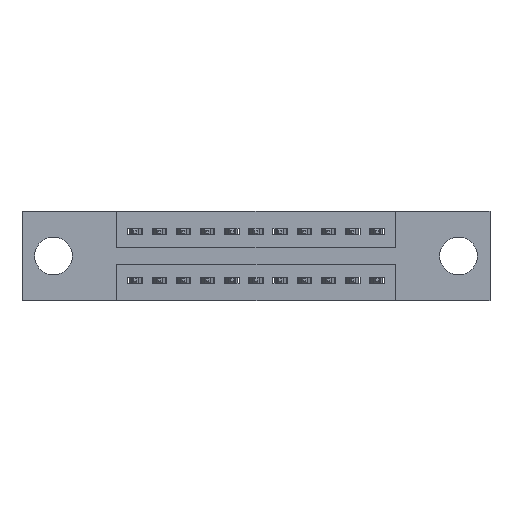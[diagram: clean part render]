
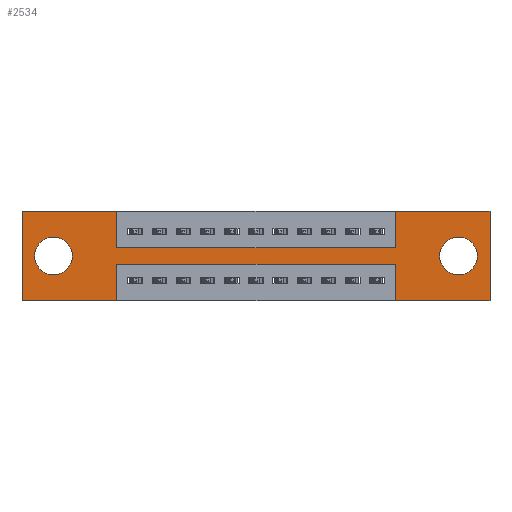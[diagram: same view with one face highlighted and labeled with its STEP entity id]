
A CAD part, front view. The second image highlights one B-rep face of the part: STEP entity #2534.
In plain terms, the highlighted planar face has unit normal (0, -1, 0).
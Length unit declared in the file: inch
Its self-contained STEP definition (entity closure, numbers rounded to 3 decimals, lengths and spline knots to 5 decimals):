
#25 = EDGE_CURVE ( 'NONE', #2283, #967, #8933, .T. ) ;
#81 = EDGE_CURVE ( 'NONE', #3398, #4703, #3219, .T. ) ;
#456 = CARTESIAN_POINT ( 'NONE',  ( 0.13, 0., -0.185 ) ) ;
#625 = EDGE_LOOP ( 'NONE', ( #5777, #4285, #12565, #6780, #1038, #3583, #9616, #1442, #11990, #6434, #9888, #9587 ) ) ;
#870 = VERTEX_POINT ( 'NONE', #12096 ) ;
#908 = VERTEX_POINT ( 'NONE', #6916 ) ;
#967 = VERTEX_POINT ( 'NONE', #8525 ) ;
#1038 = ORIENTED_EDGE ( 'NONE', *, *, #5740, .F. ) ;
#1060 = VERTEX_POINT ( 'NONE', #7505 ) ;
#1095 = ORIENTED_EDGE ( 'NONE', *, *, #81, .T. ) ;
#1110 = VERTEX_POINT ( 'NONE', #8658 ) ;
#1202 = CARTESIAN_POINT ( 'NONE',  ( 0.3925, 0., -0.22 ) ) ;
#1386 = VECTOR ( 'NONE', #11098, 39.37008 ) ;
#1394 = DIRECTION ( 'NONE',  ( 1., 0., 0. ) ) ;
#1425 = CARTESIAN_POINT ( 'NONE',  ( 1.805, 0., -0.263 ) ) ;
#1442 = ORIENTED_EDGE ( 'NONE', *, *, #12836, .F. ) ;
#1465 = CARTESIAN_POINT ( 'NONE',  ( 0., 0., -0.37 ) ) ;
#1745 = DIRECTION ( 'NONE',  ( 0., 0., 1. ) ) ;
#1771 = CARTESIAN_POINT ( 'NONE',  ( 0.13, 0., -0.107 ) ) ;
#1808 = DIRECTION ( 'NONE',  ( 0., 1., 0. ) ) ;
#1906 = DIRECTION ( 'NONE',  ( 0., 0., -1. ) ) ;
#1912 = CARTESIAN_POINT ( 'NONE',  ( 1.5425, 0., 0. ) ) ;
#1939 = VECTOR ( 'NONE', #5078, 39.37008 ) ;
#2058 = DIRECTION ( 'NONE',  ( 0., 0., -1. ) ) ;
#2173 = VECTOR ( 'NONE', #6714, 39.37008 ) ;
#2269 = VERTEX_POINT ( 'NONE', #1465 ) ;
#2283 = VERTEX_POINT ( 'NONE', #10497 ) ;
#2301 = VECTOR ( 'NONE', #5337, 39.37008 ) ;
#2317 = EDGE_CURVE ( 'NONE', #8768, #2768, #6344, .T. ) ;
#2400 = CARTESIAN_POINT ( 'NONE',  ( 0., 0., -0.37 ) ) ;
#2534 = ADVANCED_FACE ( 'NONE', ( #2786, #2661, #9044 ), #7704, .T. ) ;
#2554 = ORIENTED_EDGE ( 'NONE', *, *, #3817, .T. ) ;
#2645 = EDGE_CURVE ( 'NONE', #870, #8248, #3106, .T. ) ;
#2661 = FACE_BOUND ( 'NONE', #8489, .T. ) ;
#2666 = VECTOR ( 'NONE', #5617, 39.37008 ) ;
#2768 = VERTEX_POINT ( 'NONE', #9629 ) ;
#2786 = FACE_BOUND ( 'NONE', #13249, .T. ) ;
#2807 = VERTEX_POINT ( 'NONE', #7618 ) ;
#2918 = VECTOR ( 'NONE', #5281, 39.37008 ) ;
#3040 = DIRECTION ( 'NONE',  ( 0., -1., 0. ) ) ;
#3106 = LINE ( 'NONE', #7212, #11191 ) ;
#3219 = CIRCLE ( 'NONE', #10718, 0.078 ) ;
#3398 = VERTEX_POINT ( 'NONE', #3639 ) ;
#3556 = VERTEX_POINT ( 'NONE', #12166 ) ;
#3583 = ORIENTED_EDGE ( 'NONE', *, *, #2317, .F. ) ;
#3602 = DIRECTION ( 'NONE',  ( 0., 0., 1. ) ) ;
#3631 = CARTESIAN_POINT ( 'NONE',  ( 1.5425, 0., 0. ) ) ;
#3632 = EDGE_CURVE ( 'NONE', #4703, #3398, #5001, .T. ) ;
#3639 = CARTESIAN_POINT ( 'NONE',  ( 0.13, 0., -0.263 ) ) ;
#3731 = CARTESIAN_POINT ( 'NONE',  ( 0.3925, 0., -0.37 ) ) ;
#3768 = LINE ( 'NONE', #3631, #2173 ) ;
#3817 = EDGE_CURVE ( 'NONE', #10261, #6693, #10343, .T. ) ;
#3989 = LINE ( 'NONE', #3731, #9768 ) ;
#4172 = LINE ( 'NONE', #5308, #5423 ) ;
#4285 = ORIENTED_EDGE ( 'NONE', *, *, #7660, .F. ) ;
#4331 = CIRCLE ( 'NONE', #11868, 0.078 ) ;
#4402 = CARTESIAN_POINT ( 'NONE',  ( 0., 0., 0. ) ) ;
#4521 = EDGE_CURVE ( 'NONE', #2269, #908, #12119, .T. ) ;
#4703 = VERTEX_POINT ( 'NONE', #1771 ) ;
#4707 = CARTESIAN_POINT ( 'NONE',  ( 1.935, 0., 0. ) ) ;
#5001 = CIRCLE ( 'NONE', #9721, 0.078 ) ;
#5078 = DIRECTION ( 'NONE',  ( 0., 0., -1. ) ) ;
#5281 = DIRECTION ( 'NONE',  ( -1., 0., 0. ) ) ;
#5308 = CARTESIAN_POINT ( 'NONE',  ( 0.3925, 0., -0.15 ) ) ;
#5337 = DIRECTION ( 'NONE',  ( 1., 0., 0. ) ) ;
#5423 = VECTOR ( 'NONE', #10404, 39.37008 ) ;
#5617 = DIRECTION ( 'NONE',  ( -1., 0., 0. ) ) ;
#5740 = EDGE_CURVE ( 'NONE', #2768, #870, #6992, .T. ) ;
#5769 = DIRECTION ( 'NONE',  ( 0., 1., 0. ) ) ;
#5777 = ORIENTED_EDGE ( 'NONE', *, *, #9627, .F. ) ;
#6203 = EDGE_CURVE ( 'NONE', #8248, #2807, #11895, .T. ) ;
#6344 = LINE ( 'NONE', #12811, #2301 ) ;
#6434 = ORIENTED_EDGE ( 'NONE', *, *, #12417, .F. ) ;
#6538 = EDGE_CURVE ( 'NONE', #1060, #2269, #10577, .T. ) ;
#6693 = VERTEX_POINT ( 'NONE', #7916 ) ;
#6714 = DIRECTION ( 'NONE',  ( 0., 0., 1. ) ) ;
#6756 = CARTESIAN_POINT ( 'NONE',  ( 0., 0., -0.37 ) ) ;
#6780 = ORIENTED_EDGE ( 'NONE', *, *, #2645, .F. ) ;
#6916 = CARTESIAN_POINT ( 'NONE',  ( 0., 0., 0. ) ) ;
#6992 = LINE ( 'NONE', #4707, #7179 ) ;
#7007 = CARTESIAN_POINT ( 'NONE',  ( 0., 0., 0. ) ) ;
#7179 = VECTOR ( 'NONE', #1906, 39.37008 ) ;
#7212 = CARTESIAN_POINT ( 'NONE',  ( 0., 0., -0.37 ) ) ;
#7505 = CARTESIAN_POINT ( 'NONE',  ( 0.3925, 0., -0.37 ) ) ;
#7618 = CARTESIAN_POINT ( 'NONE',  ( 1.5425, 0., -0.22 ) ) ;
#7660 = EDGE_CURVE ( 'NONE', #2807, #3556, #10373, .T. ) ;
#7704 = PLANE ( 'NONE',  #11750 ) ;
#7916 = CARTESIAN_POINT ( 'NONE',  ( 1.805, 0., -0.107 ) ) ;
#7919 = CARTESIAN_POINT ( 'NONE',  ( 0.3925, 0., 0. ) ) ;
#8100 = DIRECTION ( 'NONE',  ( -1., 0., 0. ) ) ;
#8108 = CARTESIAN_POINT ( 'NONE',  ( 0.13, 0., -0.185 ) ) ;
#8248 = VERTEX_POINT ( 'NONE', #10907 ) ;
#8489 = EDGE_LOOP ( 'NONE', ( #11112, #1095 ) ) ;
#8525 = CARTESIAN_POINT ( 'NONE',  ( 0.3925, 0., -0.15 ) ) ;
#8644 = LINE ( 'NONE', #4402, #11875 ) ;
#8658 = CARTESIAN_POINT ( 'NONE',  ( 1.5425, 0., -0.15 ) ) ;
#8768 = VERTEX_POINT ( 'NONE', #1912 ) ;
#8875 = VECTOR ( 'NONE', #8876, 39.37008 ) ;
#8876 = DIRECTION ( 'NONE',  ( 0., 0., 1. ) ) ;
#8913 = DIRECTION ( 'NONE',  ( 0., 0., -1. ) ) ;
#8933 = LINE ( 'NONE', #7919, #1939 ) ;
#9044 = FACE_OUTER_BOUND ( 'NONE', #625, .T. ) ;
#9587 = ORIENTED_EDGE ( 'NONE', *, *, #6538, .F. ) ;
#9616 = ORIENTED_EDGE ( 'NONE', *, *, #10493, .F. ) ;
#9627 = EDGE_CURVE ( 'NONE', #3556, #1060, #3989, .T. ) ;
#9629 = CARTESIAN_POINT ( 'NONE',  ( 1.935, 0., 0. ) ) ;
#9721 = AXIS2_PLACEMENT_3D ( 'NONE', #456, #11523, #3602 ) ;
#9768 = VECTOR ( 'NONE', #8913, 39.37008 ) ;
#9859 = CARTESIAN_POINT ( 'NONE',  ( 1.5425, 0., -0.37 ) ) ;
#9888 = ORIENTED_EDGE ( 'NONE', *, *, #4521, .F. ) ;
#10261 = VERTEX_POINT ( 'NONE', #1425 ) ;
#10343 = CIRCLE ( 'NONE', #11880, 0.078 ) ;
#10373 = LINE ( 'NONE', #1202, #2918 ) ;
#10404 = DIRECTION ( 'NONE',  ( 1., 0., 0. ) ) ;
#10493 = EDGE_CURVE ( 'NONE', #1110, #8768, #3768, .T. ) ;
#10497 = CARTESIAN_POINT ( 'NONE',  ( 0.3925, 0., 0. ) ) ;
#10577 = LINE ( 'NONE', #2400, #2666 ) ;
#10718 = AXIS2_PLACEMENT_3D ( 'NONE', #8108, #1808, #1745 ) ;
#10907 = CARTESIAN_POINT ( 'NONE',  ( 1.5425, 0., -0.37 ) ) ;
#11098 = DIRECTION ( 'NONE',  ( 0., 0., 1. ) ) ;
#11109 = DIRECTION ( 'NONE',  ( 0., 0., -1. ) ) ;
#11112 = ORIENTED_EDGE ( 'NONE', *, *, #3632, .T. ) ;
#11191 = VECTOR ( 'NONE', #8100, 39.37008 ) ;
#11523 = DIRECTION ( 'NONE',  ( 0., 1., 0. ) ) ;
#11750 = AXIS2_PLACEMENT_3D ( 'NONE', #6756, #3040, #2058 ) ;
#11868 = AXIS2_PLACEMENT_3D ( 'NONE', #11888, #5769, #12079 ) ;
#11875 = VECTOR ( 'NONE', #1394, 39.37008 ) ;
#11880 = AXIS2_PLACEMENT_3D ( 'NONE', #13079, #13013, #11109 ) ;
#11888 = CARTESIAN_POINT ( 'NONE',  ( 1.805, 0., -0.185 ) ) ;
#11895 = LINE ( 'NONE', #9859, #8875 ) ;
#11990 = ORIENTED_EDGE ( 'NONE', *, *, #25, .F. ) ;
#12079 = DIRECTION ( 'NONE',  ( 0., 0., -1. ) ) ;
#12096 = CARTESIAN_POINT ( 'NONE',  ( 1.935, 0., -0.37 ) ) ;
#12119 = LINE ( 'NONE', #7007, #1386 ) ;
#12166 = CARTESIAN_POINT ( 'NONE',  ( 0.3925, 0., -0.22 ) ) ;
#12193 = ORIENTED_EDGE ( 'NONE', *, *, #12217, .T. ) ;
#12217 = EDGE_CURVE ( 'NONE', #6693, #10261, #4331, .T. ) ;
#12417 = EDGE_CURVE ( 'NONE', #908, #2283, #8644, .T. ) ;
#12565 = ORIENTED_EDGE ( 'NONE', *, *, #6203, .F. ) ;
#12811 = CARTESIAN_POINT ( 'NONE',  ( 0., 0., 0. ) ) ;
#12836 = EDGE_CURVE ( 'NONE', #967, #1110, #4172, .T. ) ;
#13013 = DIRECTION ( 'NONE',  ( 0., 1., 0. ) ) ;
#13079 = CARTESIAN_POINT ( 'NONE',  ( 1.805, 0., -0.185 ) ) ;
#13249 = EDGE_LOOP ( 'NONE', ( #12193, #2554 ) ) ;
